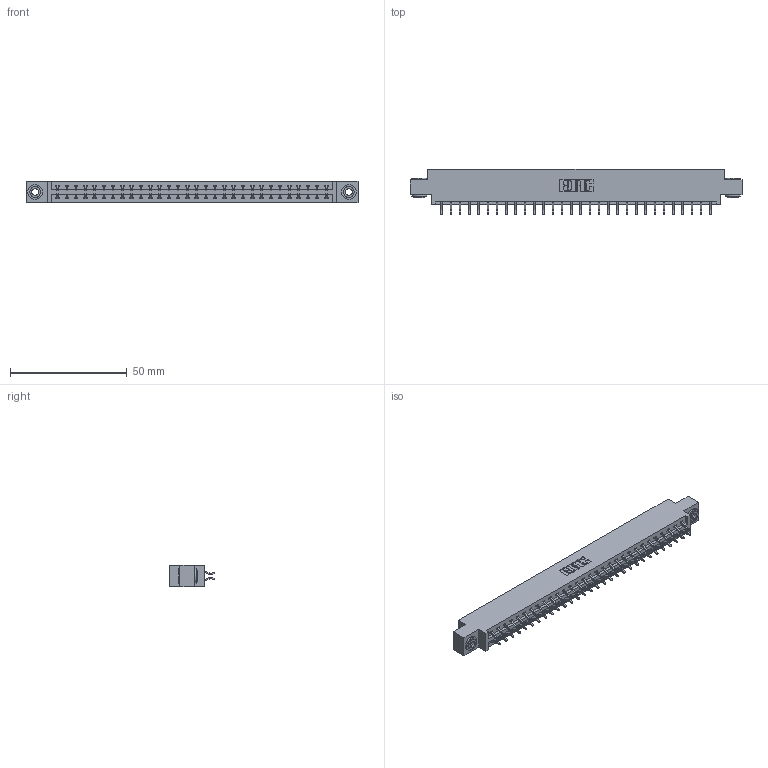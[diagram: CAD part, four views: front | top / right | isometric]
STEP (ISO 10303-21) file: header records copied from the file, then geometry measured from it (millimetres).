
FILE_DESCRIPTION (( 'STEP AP203' ), '1' );
FILE_NAME ('337-060-556-803.STEP', '2019-10-11T21:59:00', ( '' ), ( '' ), 'SwSTEP 2.0', 'SolidWorks 2016', '' );
FILE_SCHEMA (( 'CONFIG_CONTROL_DESIGN' ));
Length unit declared in the file: inch
Products named in the file (4): 337 Part_0.170 Offset - 0.156 Dia-TH; 345-292-001_556 Tail; 345-250-002_345-250-002-102; 337-060-556-803
Assembly tree (63 placements, depth 2):
  337-060-556-803
    337 Part_0.170 Offset - 0.156 Dia-TH
    345-292-001_556 Tail  x60
    345-250-002_345-250-002-102  x2
Bounding box: 141.88 x 19.57 x 9.4 mm (x, y, z)
Volume: 14692.7 mm3; surface area: 16762.5 mm2
Topology: 63 solids, 63 shells, 3756 faces, 11139 edges, 7342 vertices
Faces by surface type: plane 2604, cylinder 1144, cone 8
Entity records: 25814 total; most frequent: CARTESIAN_POINT 4349, ORIENTED_EDGE 4266, DIRECTION 3743, EDGE_CURVE 2133, VECTOR 1973, LINE 1973, VERTEX_POINT 1418, AXIS2_PLACEMENT_3D 885
